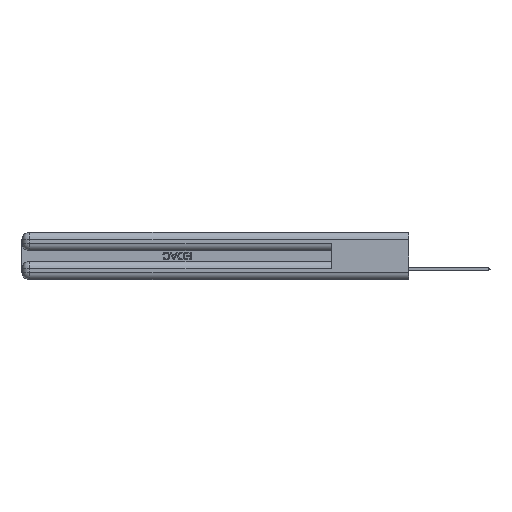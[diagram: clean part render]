
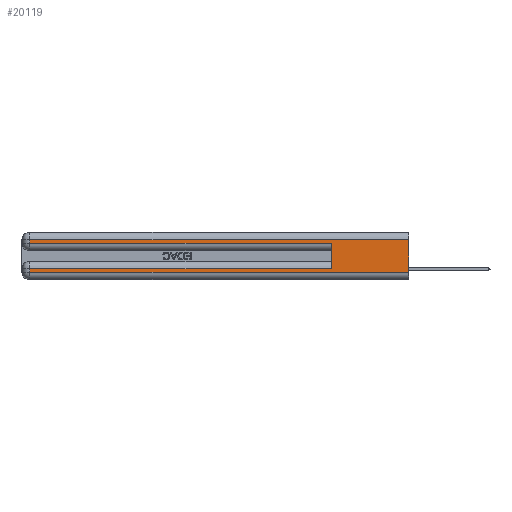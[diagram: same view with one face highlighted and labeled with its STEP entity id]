
A CAD part, left-side view. The second image highlights one B-rep face of the part: STEP entity #20119.
In plain terms, the highlighted planar face has unit normal (-1, 0, 0).
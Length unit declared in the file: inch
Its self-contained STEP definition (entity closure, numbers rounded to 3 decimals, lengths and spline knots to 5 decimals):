
#692 = CARTESIAN_POINT ( 'NONE',  ( 0., 0.6, 0.285 ) ) ;
#1391 = CARTESIAN_POINT ( 'NONE',  ( 0., 0., 0.06 ) ) ;
#1511 = DIRECTION ( 'NONE',  ( 0., 0., -1. ) ) ;
#1672 = CARTESIAN_POINT ( 'NONE',  ( 0., 2.94, 0.285 ) ) ;
#3334 = LINE ( 'NONE', #32497, #14576 ) ;
#4209 = LINE ( 'NONE', #17449, #25488 ) ;
#4825 = ORIENTED_EDGE ( 'NONE', *, *, #7024, .T. ) ;
#6085 = AXIS2_PLACEMENT_3D ( 'NONE', #33636, #9893, #1511 ) ;
#7024 = EDGE_CURVE ( 'NONE', #47210, #20195, #24245, .T. ) ;
#7118 = LINE ( 'NONE', #19987, #22150 ) ;
#8209 = VECTOR ( 'NONE', #48656, 39.37008 ) ;
#9893 = DIRECTION ( 'NONE',  ( 1., 0., 0. ) ) ;
#9967 = DIRECTION ( 'NONE',  ( 0., 0., -1. ) ) ;
#10492 = CARTESIAN_POINT ( 'NONE',  ( 0., 0., 0.37 ) ) ;
#10573 = CARTESIAN_POINT ( 'NONE',  ( 0., 0., 0.31 ) ) ;
#10918 = EDGE_CURVE ( 'NONE', #47210, #40849, #50688, .T. ) ;
#14152 = CARTESIAN_POINT ( 'NONE',  ( 0., 0.6, 0.085 ) ) ;
#14576 = VECTOR ( 'NONE', #36500, 39.37008 ) ;
#15882 = LINE ( 'NONE', #45203, #20222 ) ;
#16097 = ORIENTED_EDGE ( 'NONE', *, *, #31160, .T. ) ;
#16208 = VERTEX_POINT ( 'NONE', #1672 ) ;
#17449 = CARTESIAN_POINT ( 'NONE',  ( 0., 0., 0.285 ) ) ;
#17839 = CARTESIAN_POINT ( 'NONE',  ( 0., 2.94, 0.37 ) ) ;
#17957 = VECTOR ( 'NONE', #22334, 39.37008 ) ;
#18866 = VECTOR ( 'NONE', #38415, 39.37008 ) ;
#19987 = CARTESIAN_POINT ( 'NONE',  ( 0., 0.6, 0.145 ) ) ;
#20119 = ADVANCED_FACE ( 'NONE', ( #32154 ), #37644, .F. ) ;
#20195 = VERTEX_POINT ( 'NONE', #29638 ) ;
#20222 = VECTOR ( 'NONE', #41585, 39.37008 ) ;
#20231 = CARTESIAN_POINT ( 'NONE',  ( 0., 2.94, 0.085 ) ) ;
#22150 = VECTOR ( 'NONE', #23591, 39.37008 ) ;
#22334 = DIRECTION ( 'NONE',  ( 0., 1., 0. ) ) ;
#23591 = DIRECTION ( 'NONE',  ( 0., 0., 1. ) ) ;
#23642 = VERTEX_POINT ( 'NONE', #20231 ) ;
#23668 = VERTEX_POINT ( 'NONE', #692 ) ;
#23804 = EDGE_CURVE ( 'NONE', #16208, #23668, #4209, .T. ) ;
#24199 = ORIENTED_EDGE ( 'NONE', *, *, #10918, .F. ) ;
#24245 = LINE ( 'NONE', #10573, #17957 ) ;
#24869 = VERTEX_POINT ( 'NONE', #34053 ) ;
#25488 = VECTOR ( 'NONE', #29474, 39.37008 ) ;
#29474 = DIRECTION ( 'NONE',  ( 0., -1., 0. ) ) ;
#29638 = CARTESIAN_POINT ( 'NONE',  ( 0., 2.94, 0.31 ) ) ;
#30240 = ORIENTED_EDGE ( 'NONE', *, *, #31824, .T. ) ;
#31160 = EDGE_CURVE ( 'NONE', #20195, #16208, #3334, .T. ) ;
#31824 = EDGE_CURVE ( 'NONE', #24869, #40849, #31987, .T. ) ;
#31987 = LINE ( 'NONE', #1391, #8209 ) ;
#32154 = FACE_OUTER_BOUND ( 'NONE', #51208, .T. ) ;
#32300 = VERTEX_POINT ( 'NONE', #14152 ) ;
#32497 = CARTESIAN_POINT ( 'NONE',  ( 0., 2.94, 0.37 ) ) ;
#32539 = ORIENTED_EDGE ( 'NONE', *, *, #34453, .T. ) ;
#33636 = CARTESIAN_POINT ( 'NONE',  ( 0., 0., 0.37 ) ) ;
#34053 = CARTESIAN_POINT ( 'NONE',  ( 0., 2.94, 0.06 ) ) ;
#34453 = EDGE_CURVE ( 'NONE', #32300, #23642, #15882, .T. ) ;
#34486 = LINE ( 'NONE', #17839, #47527 ) ;
#35762 = EDGE_CURVE ( 'NONE', #23642, #24869, #34486, .T. ) ;
#36500 = DIRECTION ( 'NONE',  ( 0., 0., -1. ) ) ;
#37644 = PLANE ( 'NONE',  #6085 ) ;
#38415 = DIRECTION ( 'NONE',  ( 0., 0., -1. ) ) ;
#39995 = CARTESIAN_POINT ( 'NONE',  ( 0., 0., 0.06 ) ) ;
#40184 = ORIENTED_EDGE ( 'NONE', *, *, #44983, .F. ) ;
#40849 = VERTEX_POINT ( 'NONE', #39995 ) ;
#41585 = DIRECTION ( 'NONE',  ( 0., 1., 0. ) ) ;
#41789 = ORIENTED_EDGE ( 'NONE', *, *, #35762, .T. ) ;
#44983 = EDGE_CURVE ( 'NONE', #32300, #23668, #7118, .T. ) ;
#45203 = CARTESIAN_POINT ( 'NONE',  ( 0., 0., 0.085 ) ) ;
#46422 = CARTESIAN_POINT ( 'NONE',  ( 0., 0., 0.31 ) ) ;
#47210 = VERTEX_POINT ( 'NONE', #46422 ) ;
#47527 = VECTOR ( 'NONE', #9967, 39.37008 ) ;
#48656 = DIRECTION ( 'NONE',  ( 0., -1., 0. ) ) ;
#50130 = ORIENTED_EDGE ( 'NONE', *, *, #23804, .T. ) ;
#50688 = LINE ( 'NONE', #10492, #18866 ) ;
#51208 = EDGE_LOOP ( 'NONE', ( #24199, #4825, #16097, #50130, #40184, #32539, #41789, #30240 ) ) ;
